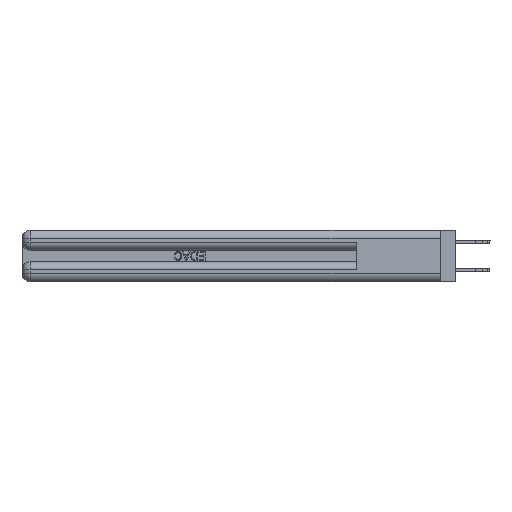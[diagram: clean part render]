
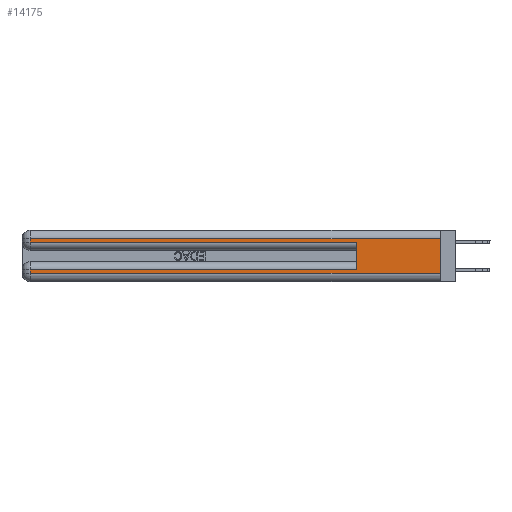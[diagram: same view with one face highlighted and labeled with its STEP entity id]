
A CAD part, left-side view. The second image highlights one B-rep face of the part: STEP entity #14175.
In plain terms, the highlighted planar face has unit normal (-1, 0, 0).
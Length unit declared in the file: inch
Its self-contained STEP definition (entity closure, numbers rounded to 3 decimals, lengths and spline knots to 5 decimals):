
#725 = DIRECTION ( 'NONE',  ( 1., 0., 0. ) ) ;
#816 = CARTESIAN_POINT ( 'NONE',  ( 0., 0.6, 0.285 ) ) ;
#865 = DIRECTION ( 'NONE',  ( 0., 0., -1. ) ) ;
#1172 = AXIS2_PLACEMENT_3D ( 'NONE', #32569, #725, #865 ) ;
#1399 = EDGE_CURVE ( 'NONE', #35853, #18634, #4332, .T. ) ;
#2122 = DIRECTION ( 'NONE',  ( 0., 0., -1. ) ) ;
#2680 = ORIENTED_EDGE ( 'NONE', *, *, #37285, .T. ) ;
#3860 = VECTOR ( 'NONE', #4191, 39.37008 ) ;
#4191 = DIRECTION ( 'NONE',  ( 0., 0., -1. ) ) ;
#4332 = LINE ( 'NONE', #11049, #26425 ) ;
#4434 = CARTESIAN_POINT ( 'NONE',  ( 0., 2.94, 0.31 ) ) ;
#4719 = ORIENTED_EDGE ( 'NONE', *, *, #35940, .T. ) ;
#4757 = CARTESIAN_POINT ( 'NONE',  ( 0., 0., 0.31 ) ) ;
#4821 = CARTESIAN_POINT ( 'NONE',  ( 0., 0.6, 0.085 ) ) ;
#5628 = CARTESIAN_POINT ( 'NONE',  ( 0., 2.94, 0.37 ) ) ;
#6270 = EDGE_CURVE ( 'NONE', #7942, #40914, #10925, .T. ) ;
#6409 = ORIENTED_EDGE ( 'NONE', *, *, #1399, .T. ) ;
#6468 = VERTEX_POINT ( 'NONE', #4434 ) ;
#7272 = LINE ( 'NONE', #13819, #21325 ) ;
#7942 = VERTEX_POINT ( 'NONE', #19989 ) ;
#8095 = DIRECTION ( 'NONE',  ( 0., -1., 0. ) ) ;
#8231 = CARTESIAN_POINT ( 'NONE',  ( 0., 0., 0.06 ) ) ;
#10164 = LINE ( 'NONE', #4757, #34737 ) ;
#10925 = LINE ( 'NONE', #16413, #3860 ) ;
#11049 = CARTESIAN_POINT ( 'NONE',  ( 0., 0., 0.285 ) ) ;
#11101 = EDGE_CURVE ( 'NONE', #19146, #18634, #7272, .T. ) ;
#11656 = EDGE_LOOP ( 'NONE', ( #35538, #2680, #25368, #6409, #25273, #4719, #35247, #18958 ) ) ;
#12347 = CARTESIAN_POINT ( 'NONE',  ( 0., 2.94, 0.285 ) ) ;
#13819 = CARTESIAN_POINT ( 'NONE',  ( 0., 0.6, 0.145 ) ) ;
#14175 = ADVANCED_FACE ( 'NONE', ( #23131 ), #29316, .F. ) ;
#14782 = DIRECTION ( 'NONE',  ( 0., 0., 1. ) ) ;
#15717 = EDGE_CURVE ( 'NONE', #6468, #35853, #38509, .T. ) ;
#16114 = DIRECTION ( 'NONE',  ( 0., 0., -1. ) ) ;
#16413 = CARTESIAN_POINT ( 'NONE',  ( 0., 2.94, 0.37 ) ) ;
#16827 = CARTESIAN_POINT ( 'NONE',  ( 0., 0., 0.31 ) ) ;
#16974 = EDGE_CURVE ( 'NONE', #41204, #39338, #22526, .T. ) ;
#18254 = CARTESIAN_POINT ( 'NONE',  ( 0., 2.94, 0.06 ) ) ;
#18634 = VERTEX_POINT ( 'NONE', #816 ) ;
#18958 = ORIENTED_EDGE ( 'NONE', *, *, #40040, .T. ) ;
#19146 = VERTEX_POINT ( 'NONE', #4821 ) ;
#19989 = CARTESIAN_POINT ( 'NONE',  ( 0., 2.94, 0.085 ) ) ;
#20148 = LINE ( 'NONE', #25648, #29610 ) ;
#21017 = VECTOR ( 'NONE', #2122, 39.37008 ) ;
#21325 = VECTOR ( 'NONE', #14782, 39.37008 ) ;
#21856 = DIRECTION ( 'NONE',  ( 0., -1., 0. ) ) ;
#22159 = CARTESIAN_POINT ( 'NONE',  ( 0., 0., 0.06 ) ) ;
#22526 = LINE ( 'NONE', #40329, #21017 ) ;
#23131 = FACE_OUTER_BOUND ( 'NONE', #11656, .T. ) ;
#25273 = ORIENTED_EDGE ( 'NONE', *, *, #11101, .F. ) ;
#25368 = ORIENTED_EDGE ( 'NONE', *, *, #15717, .T. ) ;
#25648 = CARTESIAN_POINT ( 'NONE',  ( 0., 0., 0.085 ) ) ;
#26425 = VECTOR ( 'NONE', #21856, 39.37008 ) ;
#29316 = PLANE ( 'NONE',  #1172 ) ;
#29457 = VECTOR ( 'NONE', #8095, 39.37008 ) ;
#29610 = VECTOR ( 'NONE', #31931, 39.37008 ) ;
#30517 = DIRECTION ( 'NONE',  ( 0., 1., 0. ) ) ;
#31931 = DIRECTION ( 'NONE',  ( 0., 1., 0. ) ) ;
#32569 = CARTESIAN_POINT ( 'NONE',  ( 0., 0., 0.37 ) ) ;
#34539 = LINE ( 'NONE', #8231, #29457 ) ;
#34737 = VECTOR ( 'NONE', #30517, 39.37008 ) ;
#35247 = ORIENTED_EDGE ( 'NONE', *, *, #6270, .T. ) ;
#35538 = ORIENTED_EDGE ( 'NONE', *, *, #16974, .F. ) ;
#35853 = VERTEX_POINT ( 'NONE', #12347 ) ;
#35940 = EDGE_CURVE ( 'NONE', #19146, #7942, #20148, .T. ) ;
#35993 = VECTOR ( 'NONE', #16114, 39.37008 ) ;
#37285 = EDGE_CURVE ( 'NONE', #41204, #6468, #10164, .T. ) ;
#38509 = LINE ( 'NONE', #5628, #35993 ) ;
#39338 = VERTEX_POINT ( 'NONE', #22159 ) ;
#40040 = EDGE_CURVE ( 'NONE', #40914, #39338, #34539, .T. ) ;
#40329 = CARTESIAN_POINT ( 'NONE',  ( 0., 0., 0.37 ) ) ;
#40914 = VERTEX_POINT ( 'NONE', #18254 ) ;
#41204 = VERTEX_POINT ( 'NONE', #16827 ) ;
